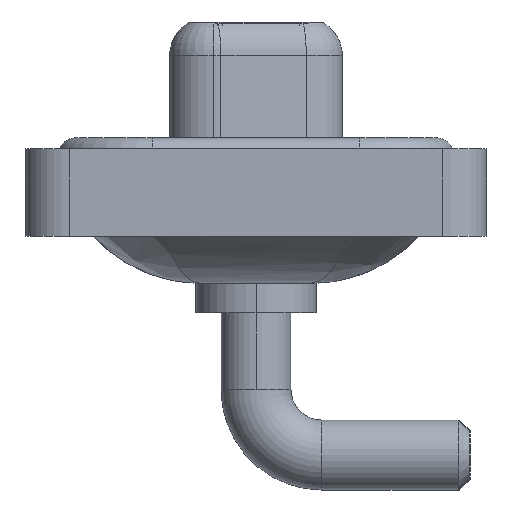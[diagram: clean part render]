
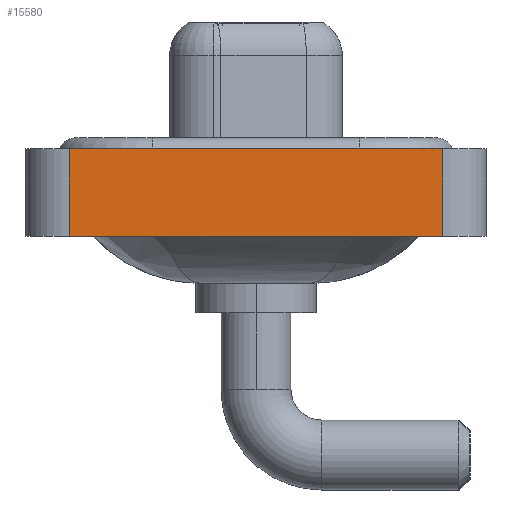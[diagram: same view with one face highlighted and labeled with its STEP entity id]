
A CAD part, left-side view. The second image highlights one B-rep face of the part: STEP entity #15580.
In plain terms, the highlighted planar face has unit normal (-1, 0, 0).
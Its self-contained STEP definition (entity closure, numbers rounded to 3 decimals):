
#113 = VECTOR ( 'NONE', #6293, 1000. ) ;
#306 = CARTESIAN_POINT ( 'NONE',  ( -7.25, -8.55, -3.6 ) ) ;
#379 = VERTEX_POINT ( 'NONE', #3923 ) ;
#778 = EDGE_CURVE ( 'NONE', #379, #931, #16303, .T. ) ;
#931 = VERTEX_POINT ( 'NONE', #306 ) ;
#2122 = DIRECTION ( 'NONE',  ( -1., 0., 0. ) ) ;
#2542 = EDGE_LOOP ( 'NONE', ( #3602, #3086, #3802, #4608 ) ) ;
#3086 = ORIENTED_EDGE ( 'NONE', *, *, #15358, .F. ) ;
#3361 = CARTESIAN_POINT ( 'NONE',  ( -7.25, -8.55, 0.4 ) ) ;
#3602 = ORIENTED_EDGE ( 'NONE', *, *, #15215, .T. ) ;
#3802 = ORIENTED_EDGE ( 'NONE', *, *, #16889, .F. ) ;
#3923 = CARTESIAN_POINT ( 'NONE',  ( -7.25, 8.55, -3.6 ) ) ;
#3982 = VECTOR ( 'NONE', #10348, 1000. ) ;
#4467 = DIRECTION ( 'NONE',  ( 0., 0., 1. ) ) ;
#4596 = CARTESIAN_POINT ( 'NONE',  ( -7.25, -8.55, -3.6 ) ) ;
#4608 = ORIENTED_EDGE ( 'NONE', *, *, #778, .T. ) ;
#5069 = LINE ( 'NONE', #6454, #113 ) ;
#6293 = DIRECTION ( 'NONE',  ( 0., 0., 1. ) ) ;
#6454 = CARTESIAN_POINT ( 'NONE',  ( -7.25, 8.55, -3.6 ) ) ;
#6962 = VERTEX_POINT ( 'NONE', #7735 ) ;
#7424 = PLANE ( 'NONE',  #12742 ) ;
#7723 = VERTEX_POINT ( 'NONE', #3361 ) ;
#7735 = CARTESIAN_POINT ( 'NONE',  ( -7.25, 8.55, 0.4 ) ) ;
#9424 = VECTOR ( 'NONE', #4467, 1000. ) ;
#9769 = LINE ( 'NONE', #11134, #9424 ) ;
#9811 = DIRECTION ( 'NONE',  ( 0., -1., 0. ) ) ;
#9903 = FACE_OUTER_BOUND ( 'NONE', #2542, .T. ) ;
#10348 = DIRECTION ( 'NONE',  ( 0., -1., 0. ) ) ;
#11134 = CARTESIAN_POINT ( 'NONE',  ( -7.25, -8.55, -3.6 ) ) ;
#11621 = LINE ( 'NONE', #11869, #3982 ) ;
#11869 = CARTESIAN_POINT ( 'NONE',  ( -7.25, -8.55, 0.4 ) ) ;
#12632 = DIRECTION ( 'NONE',  ( 0., 0., 1. ) ) ;
#12742 = AXIS2_PLACEMENT_3D ( 'NONE', #16480, #2122, #12632 ) ;
#15215 = EDGE_CURVE ( 'NONE', #931, #7723, #9769, .T. ) ;
#15358 = EDGE_CURVE ( 'NONE', #6962, #7723, #11621, .T. ) ;
#15580 = ADVANCED_FACE ( 'NONE', ( #9903 ), #7424, .T. ) ;
#15969 = VECTOR ( 'NONE', #9811, 1000. ) ;
#16303 = LINE ( 'NONE', #4596, #15969 ) ;
#16480 = CARTESIAN_POINT ( 'NONE',  ( -7.25, -8.55, -3.6 ) ) ;
#16889 = EDGE_CURVE ( 'NONE', #379, #6962, #5069, .T. ) ;
